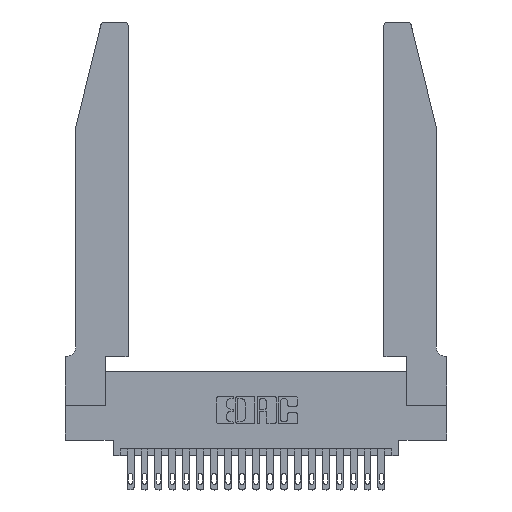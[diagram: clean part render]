
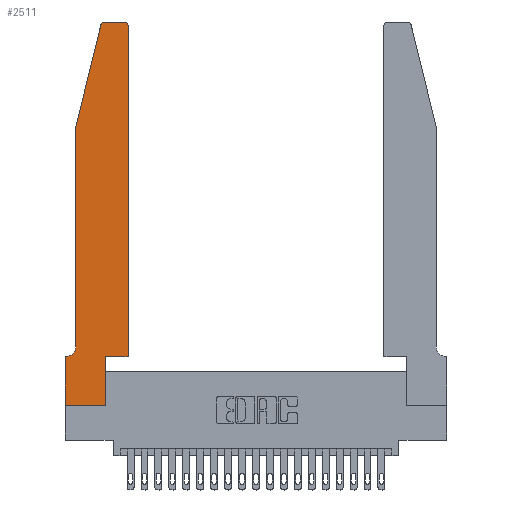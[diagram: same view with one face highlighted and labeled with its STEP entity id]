
A CAD part, top view. The second image highlights one B-rep face of the part: STEP entity #2511.
In plain terms, the highlighted planar face has unit normal (0, 0, 1).
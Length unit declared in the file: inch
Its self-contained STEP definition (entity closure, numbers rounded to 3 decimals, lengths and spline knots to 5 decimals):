
#202 = EDGE_CURVE ( 'NONE', #8028, #275, #4084, .T. ) ;
#275 = VERTEX_POINT ( 'NONE', #14130 ) ;
#517 = VERTEX_POINT ( 'NONE', #6954 ) ;
#679 = EDGE_CURVE ( 'NONE', #4131, #517, #5621, .T. ) ;
#1281 = AXIS2_PLACEMENT_3D ( 'NONE', #6293, #15506, #19310 ) ;
#1421 = CARTESIAN_POINT ( 'NONE',  ( 0.284, 2.72, 0.37 ) ) ;
#1592 = VERTEX_POINT ( 'NONE', #15031 ) ;
#2026 = CARTESIAN_POINT ( 'NONE',  ( 0., 0., 0.37 ) ) ;
#2209 = VERTEX_POINT ( 'NONE', #21322 ) ;
#2389 = CARTESIAN_POINT ( 'NONE',  ( 0.2865, 0.35, 0.37 ) ) ;
#2449 = VECTOR ( 'NONE', #10986, 39.37008 ) ;
#2511 = ADVANCED_FACE ( 'NONE', ( #7225 ), #6695, .T. ) ;
#2702 = DIRECTION ( 'NONE',  ( 1., 0., 0. ) ) ;
#3044 = CARTESIAN_POINT ( 'NONE',  ( 0.2865, 0., 0.37 ) ) ;
#3486 = DIRECTION ( 'NONE',  ( -1., 0., 0. ) ) ;
#3748 = EDGE_CURVE ( 'NONE', #1592, #4131, #22367, .T. ) ;
#4084 = LINE ( 'NONE', #8219, #7382 ) ;
#4131 = VERTEX_POINT ( 'NONE', #3044 ) ;
#4951 = VECTOR ( 'NONE', #12759, 39.37008 ) ;
#5353 = ORIENTED_EDGE ( 'NONE', *, *, #11997, .T. ) ;
#5621 = LINE ( 'NONE', #2389, #22766 ) ;
#5747 = ORIENTED_EDGE ( 'NONE', *, *, #20069, .T. ) ;
#6013 = LINE ( 'NONE', #21444, #2449 ) ;
#6149 = VERTEX_POINT ( 'NONE', #7777 ) ;
#6154 = CARTESIAN_POINT ( 'NONE',  ( 0.4205, 2.72, 0.37 ) ) ;
#6200 = ORIENTED_EDGE ( 'NONE', *, *, #9611, .T. ) ;
#6250 = VECTOR ( 'NONE', #3486, 39.37008 ) ;
#6293 = CARTESIAN_POINT ( 'NONE',  ( 0.0055, 0.42, 0.37 ) ) ;
#6695 = PLANE ( 'NONE',  #20278 ) ;
#6954 = CARTESIAN_POINT ( 'NONE',  ( 0.2865, 0.35, 0.37 ) ) ;
#7086 = CIRCLE ( 'NONE', #14291, 0.03 ) ;
#7197 = EDGE_CURVE ( 'NONE', #2209, #19625, #15156, .T. ) ;
#7225 = FACE_OUTER_BOUND ( 'NONE', #21243, .T. ) ;
#7382 = VECTOR ( 'NONE', #22317, 39.37008 ) ;
#7383 = CARTESIAN_POINT ( 'NONE',  ( 0., 0., 0.37 ) ) ;
#7484 = EDGE_CURVE ( 'NONE', #6149, #18113, #7086, .T. ) ;
#7638 = EDGE_CURVE ( 'NONE', #19625, #8108, #11234, .T. ) ;
#7777 = CARTESIAN_POINT ( 'NONE',  ( 0.284, 2.75, 0.37 ) ) ;
#7790 = DIRECTION ( 'NONE',  ( 1., 0., 0. ) ) ;
#7879 = DIRECTION ( 'NONE',  ( 0., 0., 1. ) ) ;
#8028 = VERTEX_POINT ( 'NONE', #21435 ) ;
#8108 = VERTEX_POINT ( 'NONE', #10433 ) ;
#8138 = DIRECTION ( 'NONE',  ( -0.239, -0.971, 0. ) ) ;
#8219 = CARTESIAN_POINT ( 'NONE',  ( 0.4505, 0.35, 0.37 ) ) ;
#8874 = VECTOR ( 'NONE', #17718, 39.37008 ) ;
#8948 = DIRECTION ( 'NONE',  ( 0., 0., 1. ) ) ;
#8972 = CARTESIAN_POINT ( 'NONE',  ( 0.4505, 0.35, 0.37 ) ) ;
#9123 = CIRCLE ( 'NONE', #18219, 0.03 ) ;
#9611 = EDGE_CURVE ( 'NONE', #517, #8028, #19659, .T. ) ;
#9783 = VECTOR ( 'NONE', #17747, 39.37008 ) ;
#10270 = CARTESIAN_POINT ( 'NONE',  ( 0., 0.35, 0.37 ) ) ;
#10313 = ORIENTED_EDGE ( 'NONE', *, *, #7197, .T. ) ;
#10398 = LINE ( 'NONE', #15351, #14485 ) ;
#10433 = CARTESIAN_POINT ( 'NONE',  ( 0., 0.35, 0.37 ) ) ;
#10670 = ORIENTED_EDGE ( 'NONE', *, *, #17368, .T. ) ;
#10729 = CARTESIAN_POINT ( 'NONE',  ( 0.4205, 2.75, 0.37 ) ) ;
#10818 = CARTESIAN_POINT ( 'NONE',  ( 0.0755, 0.35, 0.37 ) ) ;
#10986 = DIRECTION ( 'NONE',  ( -1., 0., 0. ) ) ;
#11047 = DIRECTION ( 'NONE',  ( 0., 1., 0. ) ) ;
#11234 = LINE ( 'NONE', #10818, #6250 ) ;
#11721 = ORIENTED_EDGE ( 'NONE', *, *, #3748, .T. ) ;
#11997 = EDGE_CURVE ( 'NONE', #15725, #2209, #17147, .T. ) ;
#12529 = DIRECTION ( 'NONE',  ( 1., 0., 0. ) ) ;
#12567 = CARTESIAN_POINT ( 'NONE',  ( 0.0755, 2., 0.37 ) ) ;
#12759 = DIRECTION ( 'NONE',  ( 0., -1., 0. ) ) ;
#14088 = EDGE_CURVE ( 'NONE', #8108, #1592, #16009, .T. ) ;
#14130 = CARTESIAN_POINT ( 'NONE',  ( 0.4505, 2.72, 0.37 ) ) ;
#14291 = AXIS2_PLACEMENT_3D ( 'NONE', #1421, #7879, #7790 ) ;
#14316 = ORIENTED_EDGE ( 'NONE', *, *, #7484, .T. ) ;
#14485 = VECTOR ( 'NONE', #8138, 39.37008 ) ;
#14654 = ORIENTED_EDGE ( 'NONE', *, *, #14088, .T. ) ;
#15031 = CARTESIAN_POINT ( 'NONE',  ( 0., 0., 0.37 ) ) ;
#15156 = CIRCLE ( 'NONE', #1281, 0.07 ) ;
#15253 = CARTESIAN_POINT ( 'NONE',  ( 0.0755, 2., 0.37 ) ) ;
#15351 = CARTESIAN_POINT ( 'NONE',  ( 0.0755, 2., 0.37 ) ) ;
#15506 = DIRECTION ( 'NONE',  ( 0., 0., -1. ) ) ;
#15725 = VERTEX_POINT ( 'NONE', #15253 ) ;
#16009 = LINE ( 'NONE', #2026, #4951 ) ;
#16664 = DIRECTION ( 'NONE',  ( 0., 0., 1. ) ) ;
#17147 = LINE ( 'NONE', #12567, #8874 ) ;
#17368 = EDGE_CURVE ( 'NONE', #18113, #15725, #10398, .T. ) ;
#17669 = VECTOR ( 'NONE', #12529, 39.37008 ) ;
#17718 = DIRECTION ( 'NONE',  ( 0., -1., 0. ) ) ;
#17747 = DIRECTION ( 'NONE',  ( 1., 0., 0. ) ) ;
#18113 = VERTEX_POINT ( 'NONE', #22590 ) ;
#18219 = AXIS2_PLACEMENT_3D ( 'NONE', #6154, #16664, #2702 ) ;
#18538 = ORIENTED_EDGE ( 'NONE', *, *, #18779, .T. ) ;
#18779 = EDGE_CURVE ( 'NONE', #275, #22358, #9123, .T. ) ;
#19310 = DIRECTION ( 'NONE',  ( -1., 0., 0. ) ) ;
#19460 = ORIENTED_EDGE ( 'NONE', *, *, #679, .T. ) ;
#19625 = VERTEX_POINT ( 'NONE', #20405 ) ;
#19659 = LINE ( 'NONE', #8972, #9783 ) ;
#20069 = EDGE_CURVE ( 'NONE', #22358, #6149, #6013, .T. ) ;
#20278 = AXIS2_PLACEMENT_3D ( 'NONE', #10270, #8948, #21258 ) ;
#20405 = CARTESIAN_POINT ( 'NONE',  ( 0.0055, 0.35, 0.37 ) ) ;
#21243 = EDGE_LOOP ( 'NONE', ( #5747, #14316, #10670, #5353, #10313, #22670, #14654, #11721, #19460, #6200, #21369, #18538 ) ) ;
#21258 = DIRECTION ( 'NONE',  ( 1., 0., 0. ) ) ;
#21322 = CARTESIAN_POINT ( 'NONE',  ( 0.0755, 0.42, 0.37 ) ) ;
#21369 = ORIENTED_EDGE ( 'NONE', *, *, #202, .T. ) ;
#21435 = CARTESIAN_POINT ( 'NONE',  ( 0.4505, 0.35, 0.37 ) ) ;
#21444 = CARTESIAN_POINT ( 'NONE',  ( 0.2605, 2.75, 0.37 ) ) ;
#22317 = DIRECTION ( 'NONE',  ( 0., 1., 0. ) ) ;
#22358 = VERTEX_POINT ( 'NONE', #10729 ) ;
#22367 = LINE ( 'NONE', #7383, #17669 ) ;
#22590 = CARTESIAN_POINT ( 'NONE',  ( 0.25487, 2.72718, 0.37 ) ) ;
#22670 = ORIENTED_EDGE ( 'NONE', *, *, #7638, .T. ) ;
#22766 = VECTOR ( 'NONE', #11047, 39.37008 ) ;
